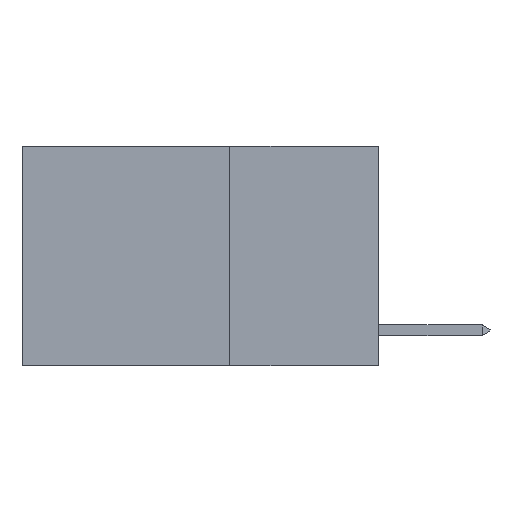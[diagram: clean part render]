
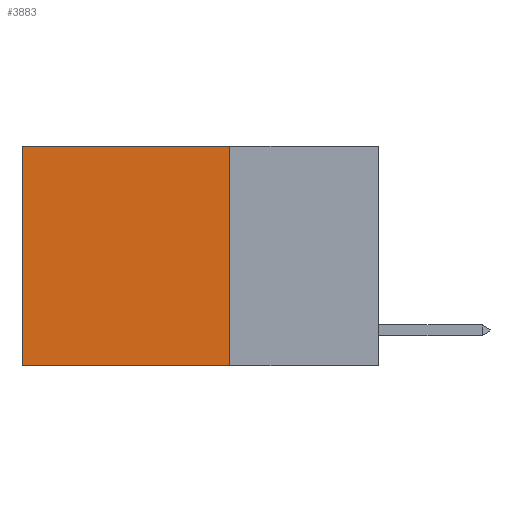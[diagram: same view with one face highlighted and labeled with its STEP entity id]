
A CAD part, left-side view. The second image highlights one B-rep face of the part: STEP entity #3883.
In plain terms, the highlighted planar face has unit normal (-1, 0, 0).
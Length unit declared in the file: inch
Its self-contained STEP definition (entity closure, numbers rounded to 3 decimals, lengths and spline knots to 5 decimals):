
#1396 = ORIENTED_EDGE ( 'NONE', *, *, #3984, .T. ) ;
#1496 = LINE ( 'NONE', #17385, #12475 ) ;
#1962 = DIRECTION ( 'NONE',  ( 0., 1., 0. ) ) ;
#2855 = VECTOR ( 'NONE', #6957, 39.37008 ) ;
#3375 = CARTESIAN_POINT ( 'NONE',  ( 0.2625, 0.6, -0.37 ) ) ;
#3883 = ADVANCED_FACE ( 'NONE', ( #5709 ), #4750, .F. ) ;
#3984 = EDGE_CURVE ( 'NONE', #9321, #7026, #13659, .T. ) ;
#4750 = PLANE ( 'NONE',  #5487 ) ;
#4907 = DIRECTION ( 'NONE',  ( 1., 0., 0. ) ) ;
#5487 = AXIS2_PLACEMENT_3D ( 'NONE', #9992, #4907, #6483 ) ;
#5709 = FACE_OUTER_BOUND ( 'NONE', #7664, .T. ) ;
#5866 = EDGE_CURVE ( 'NONE', #16129, #9321, #11487, .T. ) ;
#6098 = ORIENTED_EDGE ( 'NONE', *, *, #5866, .T. ) ;
#6483 = DIRECTION ( 'NONE',  ( 0., 0., -1. ) ) ;
#6584 = CARTESIAN_POINT ( 'NONE',  ( 0.2625, 0.25, 0. ) ) ;
#6957 = DIRECTION ( 'NONE',  ( 0., 0., -1. ) ) ;
#6999 = CARTESIAN_POINT ( 'NONE',  ( 0.2625, 0.6, 0. ) ) ;
#7026 = VERTEX_POINT ( 'NONE', #3375 ) ;
#7329 = VECTOR ( 'NONE', #12316, 39.37008 ) ;
#7664 = EDGE_LOOP ( 'NONE', ( #1396, #8335, #16101, #6098 ) ) ;
#7774 = EDGE_CURVE ( 'NONE', #11959, #7026, #10954, .T. ) ;
#8080 = CARTESIAN_POINT ( 'NONE',  ( 0.2625, 0.6, 0. ) ) ;
#8335 = ORIENTED_EDGE ( 'NONE', *, *, #7774, .F. ) ;
#8966 = CARTESIAN_POINT ( 'NONE',  ( 0.2625, 0.25, -0.37 ) ) ;
#9321 = VERTEX_POINT ( 'NONE', #8080 ) ;
#9992 = CARTESIAN_POINT ( 'NONE',  ( 0.2625, 0.25, 0. ) ) ;
#10954 = LINE ( 'NONE', #16190, #7329 ) ;
#11487 = LINE ( 'NONE', #6584, #14966 ) ;
#11959 = VERTEX_POINT ( 'NONE', #8966 ) ;
#12227 = DIRECTION ( 'NONE',  ( 0., 0., -1. ) ) ;
#12316 = DIRECTION ( 'NONE',  ( 0., 1., 0. ) ) ;
#12475 = VECTOR ( 'NONE', #12227, 39.37008 ) ;
#13659 = LINE ( 'NONE', #6999, #2855 ) ;
#14966 = VECTOR ( 'NONE', #1962, 39.37008 ) ;
#15801 = EDGE_CURVE ( 'NONE', #16129, #11959, #1496, .T. ) ;
#16101 = ORIENTED_EDGE ( 'NONE', *, *, #15801, .F. ) ;
#16129 = VERTEX_POINT ( 'NONE', #16542 ) ;
#16190 = CARTESIAN_POINT ( 'NONE',  ( 0.2625, 0.25, -0.37 ) ) ;
#16542 = CARTESIAN_POINT ( 'NONE',  ( 0.2625, 0.25, 0. ) ) ;
#17385 = CARTESIAN_POINT ( 'NONE',  ( 0.2625, 0.25, 0. ) ) ;
